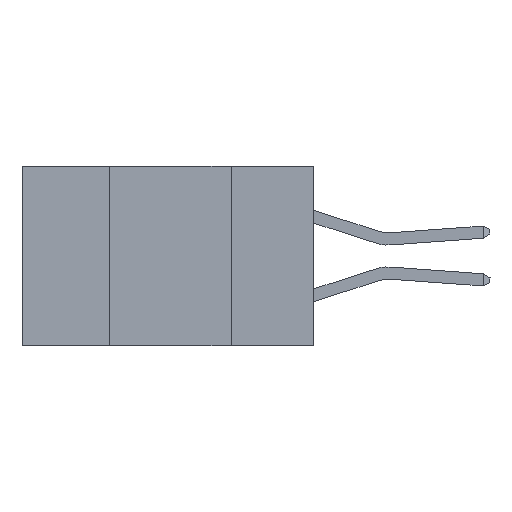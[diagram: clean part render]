
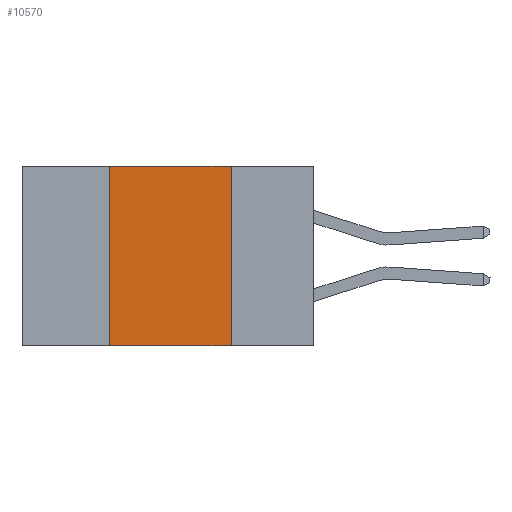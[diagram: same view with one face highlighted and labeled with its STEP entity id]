
A CAD part, left-side view. The second image highlights one B-rep face of the part: STEP entity #10570.
In plain terms, the highlighted planar face has unit normal (-1, 0, 0).
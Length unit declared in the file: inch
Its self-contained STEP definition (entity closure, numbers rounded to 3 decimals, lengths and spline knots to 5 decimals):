
#224 = VERTEX_POINT ( 'NONE', #10369 ) ;
#654 = CARTESIAN_POINT ( 'NONE',  ( 0., 0.42, 0. ) ) ;
#983 = AXIS2_PLACEMENT_3D ( 'NONE', #4737, #7319, #26566 ) ;
#1717 = EDGE_CURVE ( 'NONE', #224, #20772, #2254, .T. ) ;
#1810 = DIRECTION ( 'NONE',  ( 0., -1., 0. ) ) ;
#2254 = LINE ( 'NONE', #10245, #20786 ) ;
#2394 = LINE ( 'NONE', #7891, #27043 ) ;
#3057 = ORIENTED_EDGE ( 'NONE', *, *, #18429, .F. ) ;
#3968 = CARTESIAN_POINT ( 'NONE',  ( 0., 0.42, -0.37 ) ) ;
#4737 = CARTESIAN_POINT ( 'NONE',  ( 0., 0.6, 0. ) ) ;
#4840 = VERTEX_POINT ( 'NONE', #3968 ) ;
#5506 = DIRECTION ( 'NONE',  ( 0., -1., 0. ) ) ;
#6566 = ORIENTED_EDGE ( 'NONE', *, *, #1717, .F. ) ;
#7319 = DIRECTION ( 'NONE',  ( 1., 0., 0. ) ) ;
#7891 = CARTESIAN_POINT ( 'NONE',  ( 0., 0.6, 0. ) ) ;
#8136 = CARTESIAN_POINT ( 'NONE',  ( 0., 0.17, -0.37 ) ) ;
#8222 = ORIENTED_EDGE ( 'NONE', *, *, #28114, .F. ) ;
#8645 = ORIENTED_EDGE ( 'NONE', *, *, #17586, .T. ) ;
#10245 = CARTESIAN_POINT ( 'NONE',  ( 0., 0.17, 0. ) ) ;
#10369 = CARTESIAN_POINT ( 'NONE',  ( 0., 0.17, 0. ) ) ;
#10563 = DIRECTION ( 'NONE',  ( 0., 0., -1. ) ) ;
#10570 = ADVANCED_FACE ( 'NONE', ( #14492 ), #29245, .F. ) ;
#11538 = CARTESIAN_POINT ( 'NONE',  ( 0., 0.6, -0.37 ) ) ;
#12826 = LINE ( 'NONE', #11538, #18664 ) ;
#13877 = VECTOR ( 'NONE', #22865, 39.37008 ) ;
#14492 = FACE_OUTER_BOUND ( 'NONE', #20879, .T. ) ;
#16122 = CARTESIAN_POINT ( 'NONE',  ( 0., 0.42, 0. ) ) ;
#17586 = EDGE_CURVE ( 'NONE', #4840, #20772, #12826, .T. ) ;
#18429 = EDGE_CURVE ( 'NONE', #4840, #18590, #20417, .T. ) ;
#18590 = VERTEX_POINT ( 'NONE', #16122 ) ;
#18664 = VECTOR ( 'NONE', #1810, 39.37008 ) ;
#20417 = LINE ( 'NONE', #654, #13877 ) ;
#20772 = VERTEX_POINT ( 'NONE', #8136 ) ;
#20786 = VECTOR ( 'NONE', #10563, 39.37008 ) ;
#20879 = EDGE_LOOP ( 'NONE', ( #6566, #8222, #3057, #8645 ) ) ;
#22865 = DIRECTION ( 'NONE',  ( 0., 0., 1. ) ) ;
#26566 = DIRECTION ( 'NONE',  ( 0., 0., -1. ) ) ;
#27043 = VECTOR ( 'NONE', #5506, 39.37008 ) ;
#28114 = EDGE_CURVE ( 'NONE', #18590, #224, #2394, .T. ) ;
#29245 = PLANE ( 'NONE',  #983 ) ;
